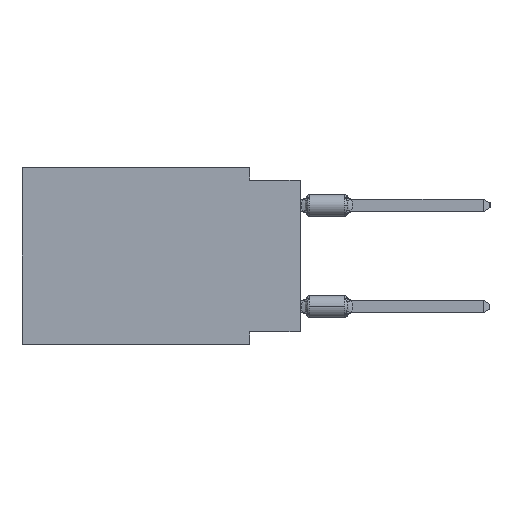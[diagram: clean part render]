
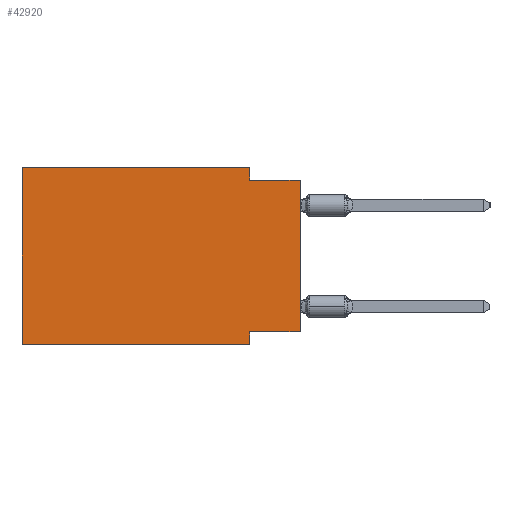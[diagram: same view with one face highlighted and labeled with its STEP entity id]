
A CAD part, left-side view. The second image highlights one B-rep face of the part: STEP entity #42920.
In plain terms, the highlighted planar face has unit normal (-1, 0, 0).
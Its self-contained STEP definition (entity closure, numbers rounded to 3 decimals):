
#215 = CARTESIAN_POINT ( 'NONE',  ( 0., 2.54, -8.255 ) ) ;
#366 = VECTOR ( 'NONE', #12382, 1000. ) ;
#764 = CARTESIAN_POINT ( 'NONE',  ( 0., 0., -8.255 ) ) ;
#998 = LINE ( 'NONE', #34718, #1591 ) ;
#1591 = VECTOR ( 'NONE', #11670, 1000. ) ;
#2668 = VECTOR ( 'NONE', #45594, 1000. ) ;
#2695 = DIRECTION ( 'NONE',  ( 0., 1., 0. ) ) ;
#3460 = DIRECTION ( 'NONE',  ( 0., 0., -1. ) ) ;
#3663 = ORIENTED_EDGE ( 'NONE', *, *, #26235, .T. ) ;
#3712 = DIRECTION ( 'NONE',  ( 1., 0., 0. ) ) ;
#4760 = LINE ( 'NONE', #7519, #12968 ) ;
#6491 = DIRECTION ( 'NONE',  ( 0., -1., 0. ) ) ;
#6952 = CARTESIAN_POINT ( 'NONE',  ( 0., 13.97, 0. ) ) ;
#7519 = CARTESIAN_POINT ( 'NONE',  ( 0., 0., -0.635 ) ) ;
#8938 = VECTOR ( 'NONE', #44874, 1000. ) ;
#9104 = VERTEX_POINT ( 'NONE', #43921 ) ;
#9455 = ORIENTED_EDGE ( 'NONE', *, *, #22395, .T. ) ;
#10790 = EDGE_CURVE ( 'NONE', #17046, #15006, #25268, .T. ) ;
#11670 = DIRECTION ( 'NONE',  ( 0., 0., -1. ) ) ;
#12181 = DIRECTION ( 'NONE',  ( 0., 0., 1. ) ) ;
#12382 = DIRECTION ( 'NONE',  ( 0., -1., 0. ) ) ;
#12838 = ORIENTED_EDGE ( 'NONE', *, *, #22008, .F. ) ;
#12968 = VECTOR ( 'NONE', #41951, 1000. ) ;
#13925 = EDGE_LOOP ( 'NONE', ( #9455, #42031, #48553, #30865, #12838, #3663, #42470, #14235 ) ) ;
#14006 = CARTESIAN_POINT ( 'NONE',  ( 0., 2.54, -8.89 ) ) ;
#14235 = ORIENTED_EDGE ( 'NONE', *, *, #10790, .F. ) ;
#15006 = VERTEX_POINT ( 'NONE', #215 ) ;
#15578 = LINE ( 'NONE', #30945, #2668 ) ;
#16421 = VERTEX_POINT ( 'NONE', #33649 ) ;
#17046 = VERTEX_POINT ( 'NONE', #764 ) ;
#18318 = LINE ( 'NONE', #45356, #8938 ) ;
#18381 = CARTESIAN_POINT ( 'NONE',  ( 0., 13.97, -8.89 ) ) ;
#19369 = VECTOR ( 'NONE', #6491, 1000. ) ;
#20059 = CARTESIAN_POINT ( 'NONE',  ( 0., 13.97, 0. ) ) ;
#20702 = VERTEX_POINT ( 'NONE', #46145 ) ;
#22008 = EDGE_CURVE ( 'NONE', #45410, #16421, #42668, .T. ) ;
#22395 = EDGE_CURVE ( 'NONE', #17046, #9104, #18318, .T. ) ;
#25268 = LINE ( 'NONE', #36661, #38713 ) ;
#25553 = EDGE_CURVE ( 'NONE', #15006, #28482, #15578, .T. ) ;
#26235 = EDGE_CURVE ( 'NONE', #45410, #28482, #30047, .T. ) ;
#28482 = VERTEX_POINT ( 'NONE', #14006 ) ;
#30047 = LINE ( 'NONE', #18381, #19369 ) ;
#30248 = PLANE ( 'NONE',  #33599 ) ;
#30865 = ORIENTED_EDGE ( 'NONE', *, *, #43123, .F. ) ;
#30945 = CARTESIAN_POINT ( 'NONE',  ( 0., 2.54, -8.89 ) ) ;
#33007 = VERTEX_POINT ( 'NONE', #43473 ) ;
#33220 = EDGE_CURVE ( 'NONE', #20702, #9104, #4760, .T. ) ;
#33599 = AXIS2_PLACEMENT_3D ( 'NONE', #6952, #3712, #3460 ) ;
#33649 = CARTESIAN_POINT ( 'NONE',  ( 0., 13.97, 0. ) ) ;
#34718 = CARTESIAN_POINT ( 'NONE',  ( 0., 2.54, 0. ) ) ;
#36135 = EDGE_CURVE ( 'NONE', #33007, #20702, #998, .T. ) ;
#36661 = CARTESIAN_POINT ( 'NONE',  ( 0., 0., -8.255 ) ) ;
#37934 = CARTESIAN_POINT ( 'NONE',  ( 0., 13.97, -8.89 ) ) ;
#38418 = LINE ( 'NONE', #20059, #366 ) ;
#38713 = VECTOR ( 'NONE', #2695, 1000. ) ;
#40919 = FACE_OUTER_BOUND ( 'NONE', #13925, .T. ) ;
#41333 = VECTOR ( 'NONE', #12181, 1000. ) ;
#41951 = DIRECTION ( 'NONE',  ( 0., -1., 0. ) ) ;
#42031 = ORIENTED_EDGE ( 'NONE', *, *, #33220, .F. ) ;
#42470 = ORIENTED_EDGE ( 'NONE', *, *, #25553, .F. ) ;
#42668 = LINE ( 'NONE', #46881, #41333 ) ;
#42920 = ADVANCED_FACE ( 'NONE', ( #40919 ), #30248, .F. ) ;
#43123 = EDGE_CURVE ( 'NONE', #16421, #33007, #38418, .T. ) ;
#43473 = CARTESIAN_POINT ( 'NONE',  ( 0., 2.54, 0. ) ) ;
#43921 = CARTESIAN_POINT ( 'NONE',  ( 0., 0., -0.635 ) ) ;
#44874 = DIRECTION ( 'NONE',  ( 0., 0., 1. ) ) ;
#45356 = CARTESIAN_POINT ( 'NONE',  ( 0., 0., 0. ) ) ;
#45410 = VERTEX_POINT ( 'NONE', #37934 ) ;
#45594 = DIRECTION ( 'NONE',  ( 0., 0., -1. ) ) ;
#46145 = CARTESIAN_POINT ( 'NONE',  ( 0., 2.54, -0.635 ) ) ;
#46881 = CARTESIAN_POINT ( 'NONE',  ( 0., 13.97, 0. ) ) ;
#48553 = ORIENTED_EDGE ( 'NONE', *, *, #36135, .F. ) ;
